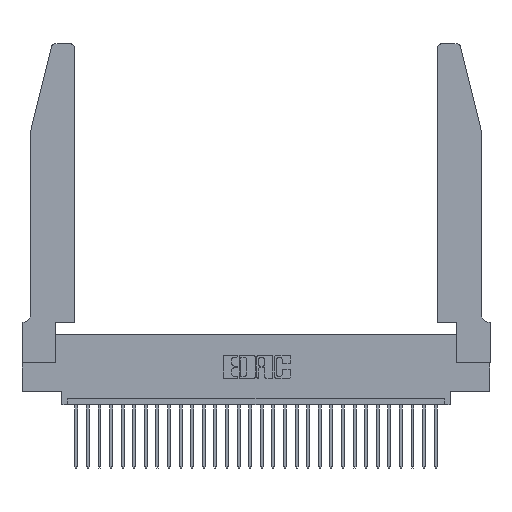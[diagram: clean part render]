
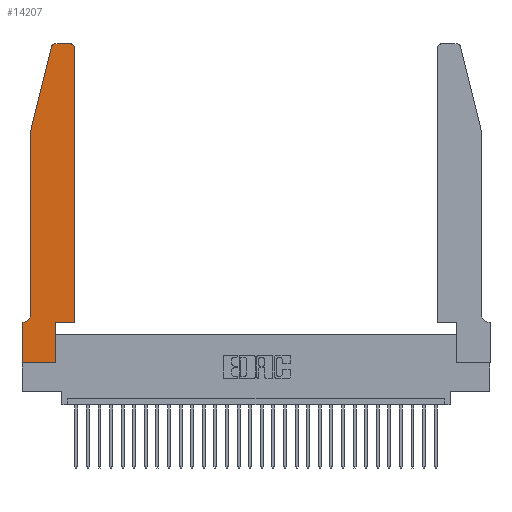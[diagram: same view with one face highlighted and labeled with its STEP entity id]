
A CAD part, top view. The second image highlights one B-rep face of the part: STEP entity #14207.
In plain terms, the highlighted planar face has unit normal (0, 0, 1).
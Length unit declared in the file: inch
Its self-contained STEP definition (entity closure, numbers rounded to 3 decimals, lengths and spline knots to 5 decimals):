
#1199 = LINE ( 'NONE', #8299, #10726 ) ;
#1501 = EDGE_CURVE ( 'NONE', #8684, #28295, #1199, .T. ) ;
#1582 = CARTESIAN_POINT ( 'NONE',  ( 0.0055, 0.42, 0.37 ) ) ;
#1748 = VECTOR ( 'NONE', #24961, 39.37008 ) ;
#2053 = CARTESIAN_POINT ( 'NONE',  ( 0.25487, 2.72718, 0.37 ) ) ;
#2269 = DIRECTION ( 'NONE',  ( 1., 0., 0. ) ) ;
#2869 = VECTOR ( 'NONE', #8040, 39.37008 ) ;
#2927 = CIRCLE ( 'NONE', #10048, 0.03 ) ;
#3005 = CARTESIAN_POINT ( 'NONE',  ( 0., 0., 0.37 ) ) ;
#3100 = CARTESIAN_POINT ( 'NONE',  ( 0., 0.35, 0.37 ) ) ;
#3832 = CARTESIAN_POINT ( 'NONE',  ( 0.2865, 0.35, 0.37 ) ) ;
#3897 = CARTESIAN_POINT ( 'NONE',  ( 0.0755, 2., 0.37 ) ) ;
#3938 = DIRECTION ( 'NONE',  ( -1., 0., 0. ) ) ;
#4590 = ORIENTED_EDGE ( 'NONE', *, *, #23094, .T. ) ;
#4800 = CARTESIAN_POINT ( 'NONE',  ( 0.0055, 0.35, 0.37 ) ) ;
#5032 = DIRECTION ( 'NONE',  ( 1., 0., 0. ) ) ;
#5076 = CARTESIAN_POINT ( 'NONE',  ( 0.4205, 2.75, 0.37 ) ) ;
#5182 = CIRCLE ( 'NONE', #13573, 0.03 ) ;
#5228 = DIRECTION ( 'NONE',  ( 0., 0., 1. ) ) ;
#5445 = DIRECTION ( 'NONE',  ( 0., 0., 1. ) ) ;
#5571 = EDGE_CURVE ( 'NONE', #29605, #23825, #17454, .T. ) ;
#5706 = CARTESIAN_POINT ( 'NONE',  ( 0.0755, 0.35, 0.37 ) ) ;
#8040 = DIRECTION ( 'NONE',  ( -1., 0., 0. ) ) ;
#8194 = EDGE_CURVE ( 'NONE', #17363, #8665, #28085, .T. ) ;
#8299 = CARTESIAN_POINT ( 'NONE',  ( 0., 0., 0.37 ) ) ;
#8665 = VERTEX_POINT ( 'NONE', #12371 ) ;
#8684 = VERTEX_POINT ( 'NONE', #26704 ) ;
#9131 = ORIENTED_EDGE ( 'NONE', *, *, #21629, .T. ) ;
#9569 = PLANE ( 'NONE',  #20880 ) ;
#10048 = AXIS2_PLACEMENT_3D ( 'NONE', #26429, #5228, #5032 ) ;
#10072 = ORIENTED_EDGE ( 'NONE', *, *, #8194, .T. ) ;
#10250 = CIRCLE ( 'NONE', #26565, 0.07 ) ;
#10574 = EDGE_CURVE ( 'NONE', #19983, #29605, #5182, .T. ) ;
#10647 = FACE_OUTER_BOUND ( 'NONE', #12303, .T. ) ;
#10703 = ORIENTED_EDGE ( 'NONE', *, *, #14362, .T. ) ;
#10726 = VECTOR ( 'NONE', #15066, 39.37008 ) ;
#11042 = ORIENTED_EDGE ( 'NONE', *, *, #10574, .T. ) ;
#11133 = CARTESIAN_POINT ( 'NONE',  ( 0.284, 2.75, 0.37 ) ) ;
#11303 = DIRECTION ( 'NONE',  ( 1., 0., 0. ) ) ;
#11949 = CARTESIAN_POINT ( 'NONE',  ( 0., 0., 0.37 ) ) ;
#11971 = VECTOR ( 'NONE', #30024, 39.37008 ) ;
#12057 = LINE ( 'NONE', #22978, #29637 ) ;
#12303 = EDGE_LOOP ( 'NONE', ( #27026, #11042, #19112, #4590, #10703, #26400, #16951, #22419, #9131, #17145, #10072, #15658 ) ) ;
#12371 = CARTESIAN_POINT ( 'NONE',  ( 0.4505, 2.72, 0.37 ) ) ;
#12429 = DIRECTION ( 'NONE',  ( 0., 1., 0. ) ) ;
#13573 = AXIS2_PLACEMENT_3D ( 'NONE', #16319, #13768, #11303 ) ;
#13768 = DIRECTION ( 'NONE',  ( 0., 0., 1. ) ) ;
#14207 = ADVANCED_FACE ( 'NONE', ( #10647 ), #9569, .T. ) ;
#14362 = EDGE_CURVE ( 'NONE', #25794, #14917, #10250, .T. ) ;
#14917 = VERTEX_POINT ( 'NONE', #4800 ) ;
#15066 = DIRECTION ( 'NONE',  ( 0., -1., 0. ) ) ;
#15329 = CARTESIAN_POINT ( 'NONE',  ( 0.2865, 0.35, 0.37 ) ) ;
#15419 = EDGE_CURVE ( 'NONE', #24564, #17363, #12057, .T. ) ;
#15658 = ORIENTED_EDGE ( 'NONE', *, *, #24926, .T. ) ;
#16222 = EDGE_CURVE ( 'NONE', #19816, #19983, #22309, .T. ) ;
#16319 = CARTESIAN_POINT ( 'NONE',  ( 0.284, 2.72, 0.37 ) ) ;
#16415 = CARTESIAN_POINT ( 'NONE',  ( 0.4505, 0.35, 0.37 ) ) ;
#16701 = LINE ( 'NONE', #21774, #26588 ) ;
#16951 = ORIENTED_EDGE ( 'NONE', *, *, #1501, .T. ) ;
#17145 = ORIENTED_EDGE ( 'NONE', *, *, #15419, .T. ) ;
#17363 = VERTEX_POINT ( 'NONE', #16415 ) ;
#17454 = LINE ( 'NONE', #3897, #11971 ) ;
#17993 = DIRECTION ( 'NONE',  ( 0., 0., -1. ) ) ;
#18113 = CARTESIAN_POINT ( 'NONE',  ( 0.0755, 0.42, 0.37 ) ) ;
#18221 = CARTESIAN_POINT ( 'NONE',  ( 0.2865, 0., 0.37 ) ) ;
#19112 = ORIENTED_EDGE ( 'NONE', *, *, #5571, .T. ) ;
#19629 = DIRECTION ( 'NONE',  ( 1., 0., 0. ) ) ;
#19816 = VERTEX_POINT ( 'NONE', #5076 ) ;
#19957 = VERTEX_POINT ( 'NONE', #18221 ) ;
#19983 = VERTEX_POINT ( 'NONE', #11133 ) ;
#20367 = EDGE_CURVE ( 'NONE', #28295, #19957, #22731, .T. ) ;
#20880 = AXIS2_PLACEMENT_3D ( 'NONE', #3100, #5445, #21846 ) ;
#21468 = VECTOR ( 'NONE', #12429, 39.37008 ) ;
#21629 = EDGE_CURVE ( 'NONE', #19957, #24564, #28523, .T. ) ;
#21774 = CARTESIAN_POINT ( 'NONE',  ( 0.0755, 2., 0.37 ) ) ;
#21846 = DIRECTION ( 'NONE',  ( 1., 0., 0. ) ) ;
#21869 = CARTESIAN_POINT ( 'NONE',  ( 0.2605, 2.75, 0.37 ) ) ;
#21892 = DIRECTION ( 'NONE',  ( -1., 0., 0. ) ) ;
#22309 = LINE ( 'NONE', #21869, #2869 ) ;
#22419 = ORIENTED_EDGE ( 'NONE', *, *, #20367, .T. ) ;
#22731 = LINE ( 'NONE', #3005, #26024 ) ;
#22978 = CARTESIAN_POINT ( 'NONE',  ( 0.4505, 0.35, 0.37 ) ) ;
#23094 = EDGE_CURVE ( 'NONE', #23825, #25794, #16701, .T. ) ;
#23825 = VERTEX_POINT ( 'NONE', #24238 ) ;
#24155 = LINE ( 'NONE', #5706, #28556 ) ;
#24238 = CARTESIAN_POINT ( 'NONE',  ( 0.0755, 2., 0.37 ) ) ;
#24564 = VERTEX_POINT ( 'NONE', #15329 ) ;
#24926 = EDGE_CURVE ( 'NONE', #8665, #19816, #2927, .T. ) ;
#24961 = DIRECTION ( 'NONE',  ( 0., 1., 0. ) ) ;
#25682 = EDGE_CURVE ( 'NONE', #14917, #8684, #24155, .T. ) ;
#25794 = VERTEX_POINT ( 'NONE', #18113 ) ;
#26024 = VECTOR ( 'NONE', #19629, 39.37008 ) ;
#26400 = ORIENTED_EDGE ( 'NONE', *, *, #25682, .T. ) ;
#26429 = CARTESIAN_POINT ( 'NONE',  ( 0.4205, 2.72, 0.37 ) ) ;
#26565 = AXIS2_PLACEMENT_3D ( 'NONE', #1582, #17993, #3938 ) ;
#26588 = VECTOR ( 'NONE', #29047, 39.37008 ) ;
#26704 = CARTESIAN_POINT ( 'NONE',  ( 0., 0.35, 0.37 ) ) ;
#27026 = ORIENTED_EDGE ( 'NONE', *, *, #16222, .T. ) ;
#28085 = LINE ( 'NONE', #29233, #21468 ) ;
#28295 = VERTEX_POINT ( 'NONE', #11949 ) ;
#28523 = LINE ( 'NONE', #3832, #1748 ) ;
#28556 = VECTOR ( 'NONE', #21892, 39.37008 ) ;
#29047 = DIRECTION ( 'NONE',  ( 0., -1., 0. ) ) ;
#29233 = CARTESIAN_POINT ( 'NONE',  ( 0.4505, 0.35, 0.37 ) ) ;
#29605 = VERTEX_POINT ( 'NONE', #2053 ) ;
#29637 = VECTOR ( 'NONE', #2269, 39.37008 ) ;
#30024 = DIRECTION ( 'NONE',  ( -0.239, -0.971, 0. ) ) ;
